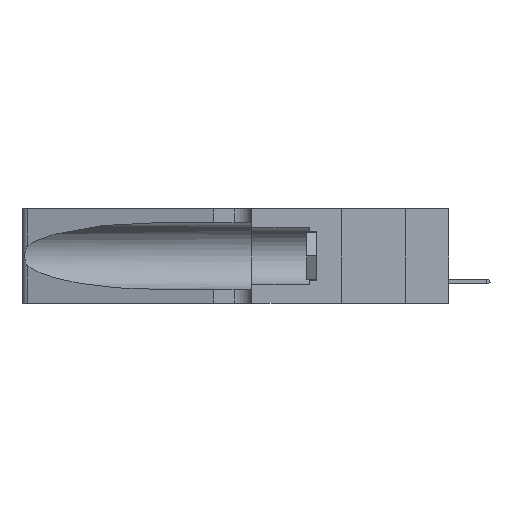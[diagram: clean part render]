
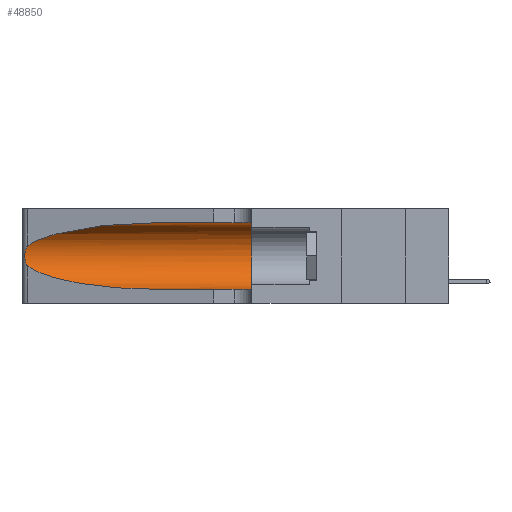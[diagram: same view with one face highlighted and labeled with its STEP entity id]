
A CAD part, left-side view. The second image highlights one B-rep face of the part: STEP entity #48850.
In plain terms, the highlighted cylindrical face has radius 3.308 mm (diameter 6.617 mm), a partial arc.
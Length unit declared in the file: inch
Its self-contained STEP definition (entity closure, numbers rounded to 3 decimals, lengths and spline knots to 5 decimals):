
#60 = VERTEX_POINT ( 'NONE', #40526 ) ;
#305 = CARTESIAN_POINT ( 'NONE',  ( 0.25856, 1.23593, 0.16098 ) ) ;
#337 = ORIENTED_EDGE ( 'NONE', *, *, #5320, .F. ) ;
#634 = EDGE_CURVE ( 'NONE', #15615, #11226, #48481, .T. ) ;
#1092 = ORIENTED_EDGE ( 'NONE', *, *, #11172, .T. ) ;
#2065 = CARTESIAN_POINT ( 'NONE',  ( 0.26075, 1.23896, 0.19203 ) ) ;
#2180 = CARTESIAN_POINT ( 'NONE',  ( 0.25487, 1.22718, 0.14631 ) ) ;
#4665 = B_SPLINE_CURVE_WITH_KNOTS ( 'NONE', 3,
 ( #34919, #46391, #47245, #32230, #39954, #32408, #2065, #48452, #34077, #305, #31636, #17017, #36376, #36715 ),
 .UNSPECIFIED., .F., .F.,
 ( 4, 2, 2, 2, 2, 2, 4 ),
 ( 0., 0.00027, 0.00053, 0.00107, 0.0016, 0.00187, 0.00214 ),
 .UNSPECIFIED. ) ;
#5320 = EDGE_CURVE ( 'NONE', #35666, #60, #44230, .T. ) ;
#6233 = FACE_OUTER_BOUND ( 'NONE', #31410, .T. ) ;
#7243 = ORIENTED_EDGE ( 'NONE', *, *, #34546, .F. ) ;
#9020 = CARTESIAN_POINT ( 'NONE',  ( 0.1305, 0.72297, 0.05475 ) ) ;
#9395 = LINE ( 'NONE', #39156, #45772 ) ;
#9921 = CARTESIAN_POINT ( 'NONE',  ( 0.2373, 1.15595, 0.08982 ) ) ;
#10362 = VERTEX_POINT ( 'NONE', #27102 ) ;
#10458 = EDGE_CURVE ( 'NONE', #11226, #60, #9395, .T. ) ;
#10835 = ORIENTED_EDGE ( 'NONE', *, *, #634, .T. ) ;
#11162 = DIRECTION ( 'NONE',  ( 0., -1., 0. ) ) ;
#11172 = EDGE_CURVE ( 'NONE', #47914, #10362, #39584, .T. ) ;
#11226 = VERTEX_POINT ( 'NONE', #9020 ) ;
#14643 = DIRECTION ( 'NONE',  ( 0., 0., -1. ) ) ;
#15615 = VERTEX_POINT ( 'NONE', #2180 ) ;
#15996 = CARTESIAN_POINT ( 'NONE',  ( 0.1305, 0.72297, 0.31525 ) ) ;
#16297 = DIRECTION ( 'NONE',  ( 0., -1., 0. ) ) ;
#17017 = CARTESIAN_POINT ( 'NONE',  ( 0.25639, 1.23186, 0.15144 ) ) ;
#17357 = VECTOR ( 'NONE', #11162, 39.37008 ) ;
#17438 = CARTESIAN_POINT ( 'NONE',  ( 0.25487, 1.22718, 0.14631 ) ) ;
#18977 = AXIS2_PLACEMENT_3D ( 'NONE', #36993, #33155, #14643 ) ;
#25786 = ORIENTED_EDGE ( 'NONE', *, *, #45135, .T. ) ;
#27102 = CARTESIAN_POINT ( 'NONE',  ( 0.25487, 1.22718, 0.22369 ) ) ;
#29640 = AXIS2_PLACEMENT_3D ( 'NONE', #42896, #38787, #42415 ) ;
#31410 = EDGE_LOOP ( 'NONE', ( #1092, #25786, #10835, #45557, #337, #7243 ) ) ;
#31636 = CARTESIAN_POINT ( 'NONE',  ( 0.25789, 1.23486, 0.15765 ) ) ;
#32230 = CARTESIAN_POINT ( 'NONE',  ( 0.25787, 1.23484, 0.2124 ) ) ;
#32264 = LINE ( 'NONE', #45186, #17357 ) ;
#32408 = CARTESIAN_POINT ( 'NONE',  ( 0.26018, 1.23835, 0.19895 ) ) ;
#32472 = CYLINDRICAL_SURFACE ( 'NONE', #18977, 0.13025 ) ;
#33155 = DIRECTION ( 'NONE',  ( 0., -1., 0. ) ) ;
#34077 = CARTESIAN_POINT ( 'NONE',  ( 0.26017, 1.23833, 0.17102 ) ) ;
#34368 = CARTESIAN_POINT ( 'NONE',  ( 0.1305, 0.35, 0.31525 ) ) ;
#34546 = EDGE_CURVE ( 'NONE', #47914, #35666, #32264, .T. ) ;
#34919 = CARTESIAN_POINT ( 'NONE',  ( 0.25487, 1.22718, 0.22369 ) ) ;
#35666 = VERTEX_POINT ( 'NONE', #34368 ) ;
#36376 = CARTESIAN_POINT ( 'NONE',  ( 0.25555, 1.22993, 0.14849 ) ) ;
#36627 = CARTESIAN_POINT ( 'NONE',  ( 0.1305, 0.72297, 0.05475 ) ) ;
#36715 = CARTESIAN_POINT ( 'NONE',  ( 0.25487, 1.22718, 0.14631 ) ) ;
#36993 = CARTESIAN_POINT ( 'NONE',  ( 0.1305, 1.61858, 0.185 ) ) ;
#37339 = CARTESIAN_POINT ( 'NONE',  ( 0.2373, 1.15595, 0.28018 ) ) ;
#38787 = DIRECTION ( 'NONE',  ( 0., 1., 0. ) ) ;
#39156 = CARTESIAN_POINT ( 'NONE',  ( 0.1305, 1.61858, 0.05475 ) ) ;
#39584 =( BOUNDED_CURVE ( )  B_SPLINE_CURVE ( 3, ( #48995, #41473, #37339, #45298 ),
 .UNSPECIFIED., .F., .F. ) 
 B_SPLINE_CURVE_WITH_KNOTS ( ( 4, 4 ),
 ( 1.5708, 2.84003 ),
 .UNSPECIFIED. ) 
 CURVE ( )  GEOMETRIC_REPRESENTATION_ITEM ( )  RATIONAL_B_SPLINE_CURVE ( ( 1., 0.87, 0.87, 1. ) ) 
 REPRESENTATION_ITEM ( '' )  );
#39954 = CARTESIAN_POINT ( 'NONE',  ( 0.25854, 1.2359, 0.20912 ) ) ;
#40526 = CARTESIAN_POINT ( 'NONE',  ( 0.1305, 0.35, 0.05475 ) ) ;
#41473 = CARTESIAN_POINT ( 'NONE',  ( 0.18966, 0.96281, 0.31525 ) ) ;
#42415 = DIRECTION ( 'NONE',  ( 0., 0., 1. ) ) ;
#42896 = CARTESIAN_POINT ( 'NONE',  ( 0.1305, 0.35, 0.185 ) ) ;
#44230 = CIRCLE ( 'NONE', #29640, 0.13025 ) ;
#45135 = EDGE_CURVE ( 'NONE', #10362, #15615, #4665, .T. ) ;
#45186 = CARTESIAN_POINT ( 'NONE',  ( 0.1305, 1.61858, 0.31525 ) ) ;
#45298 = CARTESIAN_POINT ( 'NONE',  ( 0.25487, 1.22718, 0.22369 ) ) ;
#45557 = ORIENTED_EDGE ( 'NONE', *, *, #10458, .T. ) ;
#45772 = VECTOR ( 'NONE', #16297, 39.37008 ) ;
#46391 = CARTESIAN_POINT ( 'NONE',  ( 0.25555, 1.22994, 0.2215 ) ) ;
#47245 = CARTESIAN_POINT ( 'NONE',  ( 0.25639, 1.23184, 0.21858 ) ) ;
#47914 = VERTEX_POINT ( 'NONE', #15996 ) ;
#47953 = CARTESIAN_POINT ( 'NONE',  ( 0.18966, 0.96281, 0.05475 ) ) ;
#48452 = CARTESIAN_POINT ( 'NONE',  ( 0.26075, 1.23896, 0.178 ) ) ;
#48481 =( BOUNDED_CURVE ( )  B_SPLINE_CURVE ( 3, ( #17438, #9921, #47953, #36627 ),
 .UNSPECIFIED., .F., .F. ) 
 B_SPLINE_CURVE_WITH_KNOTS ( ( 4, 4 ),
 ( 3.44316, 4.71239 ),
 .UNSPECIFIED. ) 
 CURVE ( )  GEOMETRIC_REPRESENTATION_ITEM ( )  RATIONAL_B_SPLINE_CURVE ( ( 1., 0.87, 0.87, 1. ) ) 
 REPRESENTATION_ITEM ( '' )  );
#48850 = ADVANCED_FACE ( 'NONE', ( #6233 ), #32472, .F. ) ;
#48995 = CARTESIAN_POINT ( 'NONE',  ( 0.1305, 0.72297, 0.31525 ) ) ;
